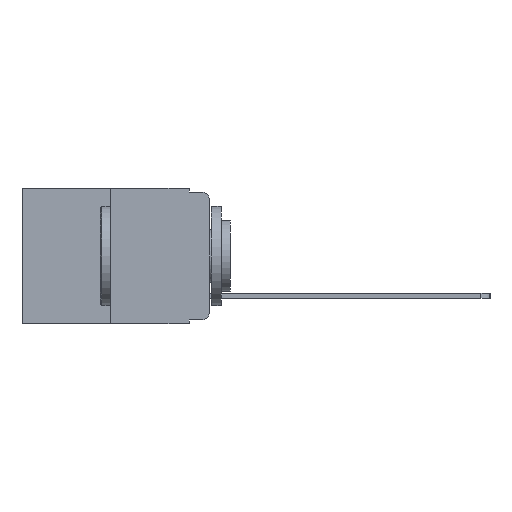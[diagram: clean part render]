
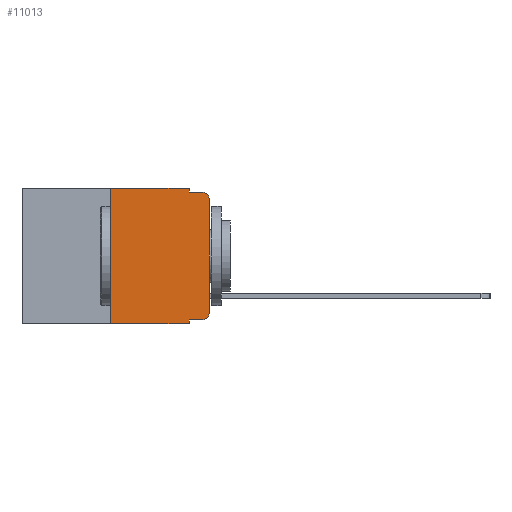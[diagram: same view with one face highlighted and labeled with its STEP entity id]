
A CAD part, left-side view. The second image highlights one B-rep face of the part: STEP entity #11013.
In plain terms, the highlighted planar face has unit normal (-1, 0, 0).
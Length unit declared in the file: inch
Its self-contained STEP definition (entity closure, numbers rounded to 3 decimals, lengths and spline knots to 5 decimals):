
#222 = CARTESIAN_POINT ( 'NONE',  ( 0., 0.051, 0. ) ) ;
#348 = LINE ( 'NONE', #13511, #12355 ) ;
#1236 = ORIENTED_EDGE ( 'NONE', *, *, #15245, .T. ) ;
#1720 = CIRCLE ( 'NONE', #19572, 0.02 ) ;
#2006 = ORIENTED_EDGE ( 'NONE', *, *, #16603, .T. ) ;
#2111 = CARTESIAN_POINT ( 'NONE',  ( 0., 0.02, -0.333 ) ) ;
#2218 = EDGE_CURVE ( 'NONE', #2655, #19860, #9299, .T. ) ;
#2315 = VERTEX_POINT ( 'NONE', #7883 ) ;
#2439 = CIRCLE ( 'NONE', #11254, 0.02 ) ;
#2515 = CARTESIAN_POINT ( 'NONE',  ( 0., 0.473, 0. ) ) ;
#2543 = LINE ( 'NONE', #15906, #9905 ) ;
#2587 = CARTESIAN_POINT ( 'NONE',  ( 0., 0.051, 0. ) ) ;
#2655 = VERTEX_POINT ( 'NONE', #2969 ) ;
#2692 = FACE_OUTER_BOUND ( 'NONE', #10409, .T. ) ;
#2856 = VERTEX_POINT ( 'NONE', #7335 ) ;
#2969 = CARTESIAN_POINT ( 'NONE',  ( 0., 0.25, 0. ) ) ;
#3170 = CARTESIAN_POINT ( 'NONE',  ( 0., 0.051, -0.01 ) ) ;
#3217 = ORIENTED_EDGE ( 'NONE', *, *, #7120, .F. ) ;
#3683 = VECTOR ( 'NONE', #9411, 39.37008 ) ;
#3714 = ORIENTED_EDGE ( 'NONE', *, *, #2218, .F. ) ;
#3733 = LINE ( 'NONE', #9302, #15961 ) ;
#3911 = EDGE_CURVE ( 'NONE', #16221, #2655, #6079, .T. ) ;
#5248 = DIRECTION ( 'NONE',  ( 0., 0., -1. ) ) ;
#5461 = VERTEX_POINT ( 'NONE', #16351 ) ;
#5488 = VECTOR ( 'NONE', #16904, 39.37008 ) ;
#6071 = CARTESIAN_POINT ( 'NONE',  ( 0., 0.02, -0.03 ) ) ;
#6079 = LINE ( 'NONE', #9593, #10197 ) ;
#6467 = ORIENTED_EDGE ( 'NONE', *, *, #11256, .T. ) ;
#6563 = CARTESIAN_POINT ( 'NONE',  ( 0., 0.02, -0.313 ) ) ;
#7043 = DIRECTION ( 'NONE',  ( 0., 0., -1. ) ) ;
#7120 = EDGE_CURVE ( 'NONE', #19860, #9973, #10833, .T. ) ;
#7335 = CARTESIAN_POINT ( 'NONE',  ( 0., 0.02, -0.01 ) ) ;
#7644 = DIRECTION ( 'NONE',  ( 0., 0., -1. ) ) ;
#7883 = CARTESIAN_POINT ( 'NONE',  ( 0., 0., -0.03 ) ) ;
#8115 = DIRECTION ( 'NONE',  ( 0., 0., -1. ) ) ;
#8145 = EDGE_CURVE ( 'NONE', #9973, #2856, #19439, .T. ) ;
#8512 = PLANE ( 'NONE',  #14625 ) ;
#8589 = CARTESIAN_POINT ( 'NONE',  ( 0., 0.25, -0.343 ) ) ;
#8856 = ORIENTED_EDGE ( 'NONE', *, *, #8884, .T. ) ;
#8884 = EDGE_CURVE ( 'NONE', #16221, #5461, #17626, .T. ) ;
#9299 = LINE ( 'NONE', #2515, #17764 ) ;
#9302 = CARTESIAN_POINT ( 'NONE',  ( 0., 0., 0. ) ) ;
#9411 = DIRECTION ( 'NONE',  ( 0., -1., 0. ) ) ;
#9593 = CARTESIAN_POINT ( 'NONE',  ( 0., 0.25, 0. ) ) ;
#9640 = DIRECTION ( 'NONE',  ( 0., -1., 0. ) ) ;
#9905 = VECTOR ( 'NONE', #5248, 39.37008 ) ;
#9973 = VERTEX_POINT ( 'NONE', #14835 ) ;
#10197 = VECTOR ( 'NONE', #18590, 39.37008 ) ;
#10409 = EDGE_LOOP ( 'NONE', ( #1236, #6467, #15022, #3217, #3714, #12499, #8856, #16897, #13395, #2006 ) ) ;
#10833 = LINE ( 'NONE', #222, #18302 ) ;
#11013 = ADVANCED_FACE ( 'NONE', ( #2692 ), #8512, .F. ) ;
#11254 = AXIS2_PLACEMENT_3D ( 'NONE', #6071, #16675, #7644 ) ;
#11256 = EDGE_CURVE ( 'NONE', #2315, #2856, #2439, .T. ) ;
#11550 = VERTEX_POINT ( 'NONE', #2111 ) ;
#12355 = VECTOR ( 'NONE', #16420, 39.37008 ) ;
#12499 = ORIENTED_EDGE ( 'NONE', *, *, #3911, .F. ) ;
#13293 = VERTEX_POINT ( 'NONE', #15904 ) ;
#13395 = ORIENTED_EDGE ( 'NONE', *, *, #18623, .T. ) ;
#13511 = CARTESIAN_POINT ( 'NONE',  ( 0., 0.051, -0.333 ) ) ;
#14617 = CARTESIAN_POINT ( 'NONE',  ( 0., 0.473, 0. ) ) ;
#14625 = AXIS2_PLACEMENT_3D ( 'NONE', #14617, #16095, #7043 ) ;
#14835 = CARTESIAN_POINT ( 'NONE',  ( 0., 0.051, -0.01 ) ) ;
#15022 = ORIENTED_EDGE ( 'NONE', *, *, #8145, .F. ) ;
#15245 = EDGE_CURVE ( 'NONE', #19295, #2315, #3733, .T. ) ;
#15398 = CARTESIAN_POINT ( 'NONE',  ( 0., 0.473, -0.343 ) ) ;
#15707 = DIRECTION ( 'NONE',  ( 0., 0., -1. ) ) ;
#15904 = CARTESIAN_POINT ( 'NONE',  ( 0., 0.051, -0.333 ) ) ;
#15906 = CARTESIAN_POINT ( 'NONE',  ( 0., 0.051, 0. ) ) ;
#15961 = VECTOR ( 'NONE', #19833, 39.37008 ) ;
#16095 = DIRECTION ( 'NONE',  ( 1., 0., 0. ) ) ;
#16221 = VERTEX_POINT ( 'NONE', #8589 ) ;
#16351 = CARTESIAN_POINT ( 'NONE',  ( 0., 0.051, -0.343 ) ) ;
#16420 = DIRECTION ( 'NONE',  ( 0., -1., 0. ) ) ;
#16603 = EDGE_CURVE ( 'NONE', #11550, #19295, #1720, .T. ) ;
#16675 = DIRECTION ( 'NONE',  ( -1., 0., 0. ) ) ;
#16897 = ORIENTED_EDGE ( 'NONE', *, *, #19634, .F. ) ;
#16904 = DIRECTION ( 'NONE',  ( 0., -1., 0. ) ) ;
#17151 = DIRECTION ( 'NONE',  ( -1., 0., 0. ) ) ;
#17626 = LINE ( 'NONE', #15398, #5488 ) ;
#17764 = VECTOR ( 'NONE', #9640, 39.37008 ) ;
#18074 = CARTESIAN_POINT ( 'NONE',  ( 0., 0., -0.313 ) ) ;
#18302 = VECTOR ( 'NONE', #15707, 39.37008 ) ;
#18590 = DIRECTION ( 'NONE',  ( 0., 0., 1. ) ) ;
#18623 = EDGE_CURVE ( 'NONE', #13293, #11550, #348, .T. ) ;
#19295 = VERTEX_POINT ( 'NONE', #18074 ) ;
#19439 = LINE ( 'NONE', #3170, #3683 ) ;
#19572 = AXIS2_PLACEMENT_3D ( 'NONE', #6563, #17151, #8115 ) ;
#19634 = EDGE_CURVE ( 'NONE', #13293, #5461, #2543, .T. ) ;
#19833 = DIRECTION ( 'NONE',  ( 0., 0., 1. ) ) ;
#19860 = VERTEX_POINT ( 'NONE', #2587 ) ;
